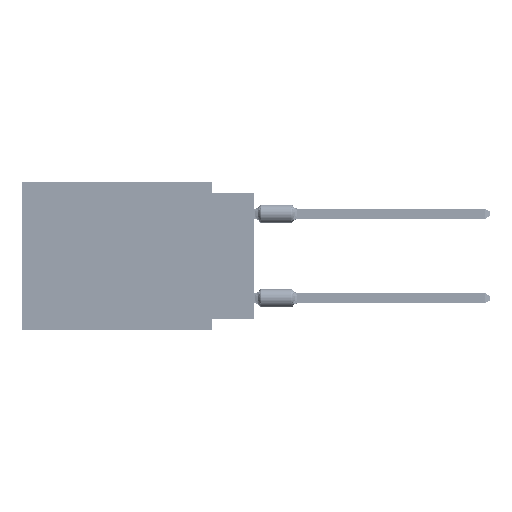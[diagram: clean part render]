
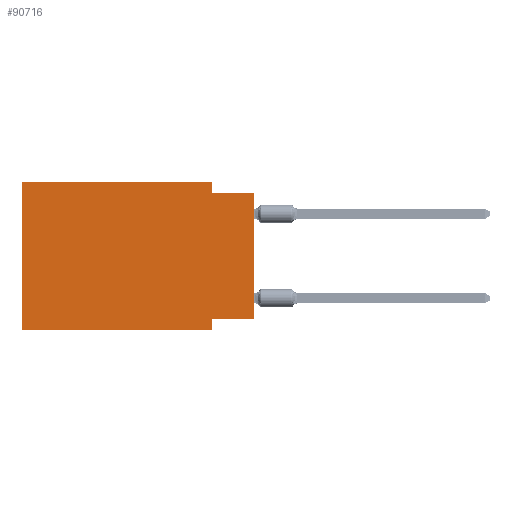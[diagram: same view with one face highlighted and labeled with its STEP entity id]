
A CAD part, left-side view. The second image highlights one B-rep face of the part: STEP entity #90716.
In plain terms, the highlighted planar face has unit normal (-1, 0, 0).
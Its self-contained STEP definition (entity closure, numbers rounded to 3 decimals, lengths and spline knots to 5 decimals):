
#637 = LINE ( 'NONE', #1223, #16025 ) ;
#1223 = CARTESIAN_POINT ( 'NONE',  ( 0., 0.1, -0.35 ) ) ;
#4345 = LINE ( 'NONE', #12742, #77692 ) ;
#12742 = CARTESIAN_POINT ( 'NONE',  ( 0., 0., 0. ) ) ;
#12819 = CARTESIAN_POINT ( 'NONE',  ( 0., 0.55, 0. ) ) ;
#16025 = VECTOR ( 'NONE', #38988, 39.37008 ) ;
#16831 = DIRECTION ( 'NONE',  ( 0., 0., -1. ) ) ;
#17428 = PLANE ( 'NONE',  #113263 ) ;
#17566 = CARTESIAN_POINT ( 'NONE',  ( 0., 0.1, -0.325 ) ) ;
#18767 = ORIENTED_EDGE ( 'NONE', *, *, #59188, .F. ) ;
#19300 = LINE ( 'NONE', #54705, #59938 ) ;
#21009 = DIRECTION ( 'NONE',  ( 0., 0., -1. ) ) ;
#22205 = LINE ( 'NONE', #85223, #42379 ) ;
#22341 = DIRECTION ( 'NONE',  ( 0., 0., 1. ) ) ;
#23585 = CARTESIAN_POINT ( 'NONE',  ( 0., 0.1, 0. ) ) ;
#25841 = CARTESIAN_POINT ( 'NONE',  ( 0., 0.55, 0. ) ) ;
#26156 = VERTEX_POINT ( 'NONE', #57533 ) ;
#28394 = ORIENTED_EDGE ( 'NONE', *, *, #31298, .F. ) ;
#29633 = LINE ( 'NONE', #38634, #50925 ) ;
#29938 = VERTEX_POINT ( 'NONE', #71579 ) ;
#30705 = DIRECTION ( 'NONE',  ( 0., 0., 1. ) ) ;
#31098 = DIRECTION ( 'NONE',  ( 0., 1., 0. ) ) ;
#31298 = EDGE_CURVE ( 'NONE', #46284, #41901, #19300, .T. ) ;
#31429 = DIRECTION ( 'NONE',  ( 0., -1., 0. ) ) ;
#31880 = CARTESIAN_POINT ( 'NONE',  ( 0., 0.55, 0. ) ) ;
#35052 = EDGE_CURVE ( 'NONE', #104228, #86329, #29633, .T. ) ;
#37045 = EDGE_CURVE ( 'NONE', #29938, #46284, #76308, .T. ) ;
#38634 = CARTESIAN_POINT ( 'NONE',  ( 0., 0., -0.025 ) ) ;
#38988 = DIRECTION ( 'NONE',  ( 0., 0., -1. ) ) ;
#40084 = LINE ( 'NONE', #103710, #91068 ) ;
#40728 = ORIENTED_EDGE ( 'NONE', *, *, #37045, .F. ) ;
#41281 = VECTOR ( 'NONE', #82711, 39.37008 ) ;
#41807 = ORIENTED_EDGE ( 'NONE', *, *, #82469, .F. ) ;
#41901 = VERTEX_POINT ( 'NONE', #23585 ) ;
#42379 = VECTOR ( 'NONE', #21009, 39.37008 ) ;
#46284 = VERTEX_POINT ( 'NONE', #12819 ) ;
#50925 = VECTOR ( 'NONE', #31429, 39.37008 ) ;
#54705 = CARTESIAN_POINT ( 'NONE',  ( 0., 0.55, 0. ) ) ;
#57533 = CARTESIAN_POINT ( 'NONE',  ( 0., 0., -0.325 ) ) ;
#59188 = EDGE_CURVE ( 'NONE', #41901, #104228, #22205, .T. ) ;
#59938 = VECTOR ( 'NONE', #83501, 39.37008 ) ;
#60656 = FACE_OUTER_BOUND ( 'NONE', #66453, .T. ) ;
#62440 = DIRECTION ( 'NONE',  ( 1., 0., 0. ) ) ;
#66453 = EDGE_LOOP ( 'NONE', ( #101611, #71367, #18767, #28394, #40728, #73465, #79843, #41807 ) ) ;
#71367 = ORIENTED_EDGE ( 'NONE', *, *, #35052, .F. ) ;
#71579 = CARTESIAN_POINT ( 'NONE',  ( 0., 0.55, -0.35 ) ) ;
#72526 = LINE ( 'NONE', #100730, #41281 ) ;
#73047 = EDGE_CURVE ( 'NONE', #29938, #78506, #72526, .T. ) ;
#73465 = ORIENTED_EDGE ( 'NONE', *, *, #73047, .T. ) ;
#76308 = LINE ( 'NONE', #31880, #110406 ) ;
#77692 = VECTOR ( 'NONE', #22341, 39.37008 ) ;
#78506 = VERTEX_POINT ( 'NONE', #95368 ) ;
#79439 = EDGE_CURVE ( 'NONE', #107670, #78506, #637, .T. ) ;
#79843 = ORIENTED_EDGE ( 'NONE', *, *, #79439, .F. ) ;
#82469 = EDGE_CURVE ( 'NONE', #26156, #107670, #40084, .T. ) ;
#82711 = DIRECTION ( 'NONE',  ( 0., -1., 0. ) ) ;
#83501 = DIRECTION ( 'NONE',  ( 0., -1., 0. ) ) ;
#85223 = CARTESIAN_POINT ( 'NONE',  ( 0., 0.1, 0. ) ) ;
#86329 = VERTEX_POINT ( 'NONE', #98690 ) ;
#90716 = ADVANCED_FACE ( 'NONE', ( #60656 ), #17428, .F. ) ;
#91068 = VECTOR ( 'NONE', #31098, 39.37008 ) ;
#95368 = CARTESIAN_POINT ( 'NONE',  ( 0., 0.1, -0.35 ) ) ;
#95687 = CARTESIAN_POINT ( 'NONE',  ( 0., 0.1, -0.025 ) ) ;
#96784 = EDGE_CURVE ( 'NONE', #26156, #86329, #4345, .T. ) ;
#98690 = CARTESIAN_POINT ( 'NONE',  ( 0., 0., -0.025 ) ) ;
#100730 = CARTESIAN_POINT ( 'NONE',  ( 0., 0.55, -0.35 ) ) ;
#101611 = ORIENTED_EDGE ( 'NONE', *, *, #96784, .T. ) ;
#103710 = CARTESIAN_POINT ( 'NONE',  ( 0., 0., -0.325 ) ) ;
#104228 = VERTEX_POINT ( 'NONE', #95687 ) ;
#107670 = VERTEX_POINT ( 'NONE', #17566 ) ;
#110406 = VECTOR ( 'NONE', #30705, 39.37008 ) ;
#113263 = AXIS2_PLACEMENT_3D ( 'NONE', #25841, #62440, #16831 ) ;
